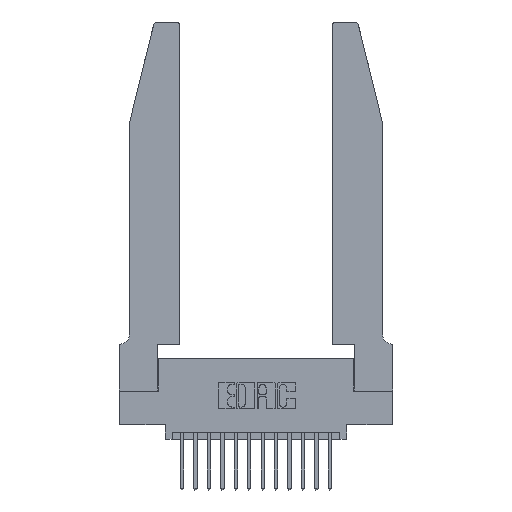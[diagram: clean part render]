
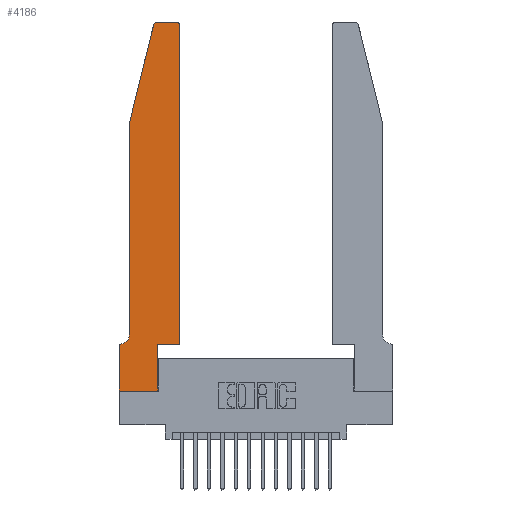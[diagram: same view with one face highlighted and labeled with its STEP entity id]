
A CAD part, top view. The second image highlights one B-rep face of the part: STEP entity #4186.
In plain terms, the highlighted planar face has unit normal (0, 0, 1).
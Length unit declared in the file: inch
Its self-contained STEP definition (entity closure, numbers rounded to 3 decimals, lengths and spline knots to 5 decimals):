
#68 = ORIENTED_EDGE ( 'NONE', *, *, #2993, .T. ) ;
#72 = CARTESIAN_POINT ( 'NONE',  ( 0.284, 2.75, 0.37 ) ) ;
#155 = EDGE_CURVE ( 'NONE', #11812, #13700, #17308, .T. ) ;
#1201 = EDGE_CURVE ( 'NONE', #9545, #7167, #5894, .T. ) ;
#1401 = LINE ( 'NONE', #8634, #16089 ) ;
#1418 = DIRECTION ( 'NONE',  ( 0., 0., 1. ) ) ;
#1608 = DIRECTION ( 'NONE',  ( 1., 0., 0. ) ) ;
#1954 = VECTOR ( 'NONE', #7813, 39.37008 ) ;
#1973 = VERTEX_POINT ( 'NONE', #15770 ) ;
#2091 = CARTESIAN_POINT ( 'NONE',  ( 0.0755, 0.35, 0.37 ) ) ;
#2262 = CARTESIAN_POINT ( 'NONE',  ( 0.4205, 2.75, 0.37 ) ) ;
#2316 = VERTEX_POINT ( 'NONE', #3792 ) ;
#2352 = CARTESIAN_POINT ( 'NONE',  ( 0.2865, 0., 0.37 ) ) ;
#2741 = DIRECTION ( 'NONE',  ( 0., 0., 1. ) ) ;
#2993 = EDGE_CURVE ( 'NONE', #6156, #1973, #8489, .T. ) ;
#3792 = CARTESIAN_POINT ( 'NONE',  ( 0.4505, 0.35, 0.37 ) ) ;
#3988 = VERTEX_POINT ( 'NONE', #17971 ) ;
#4166 = LINE ( 'NONE', #10574, #17501 ) ;
#4186 = ADVANCED_FACE ( 'NONE', ( #4870 ), #15073, .T. ) ;
#4292 = CARTESIAN_POINT ( 'NONE',  ( 0.4505, 2.72, 0.37 ) ) ;
#4484 = DIRECTION ( 'NONE',  ( 0., 0., -1. ) ) ;
#4489 = VECTOR ( 'NONE', #5891, 39.37008 ) ;
#4744 = AXIS2_PLACEMENT_3D ( 'NONE', #12536, #12012, #8576 ) ;
#4860 = ORIENTED_EDGE ( 'NONE', *, *, #15753, .T. ) ;
#4870 = FACE_OUTER_BOUND ( 'NONE', #14786, .T. ) ;
#5052 = ORIENTED_EDGE ( 'NONE', *, *, #17736, .T. ) ;
#5061 = VECTOR ( 'NONE', #9549, 39.37008 ) ;
#5888 = DIRECTION ( 'NONE',  ( -1., 0., 0. ) ) ;
#5891 = DIRECTION ( 'NONE',  ( 0., 1., 0. ) ) ;
#5894 = CIRCLE ( 'NONE', #4744, 0.03 ) ;
#5960 = VERTEX_POINT ( 'NONE', #13731 ) ;
#6041 = LINE ( 'NONE', #13011, #17624 ) ;
#6156 = VERTEX_POINT ( 'NONE', #72 ) ;
#6267 = EDGE_CURVE ( 'NONE', #13700, #17199, #4166, .T. ) ;
#6465 = DIRECTION ( 'NONE',  ( -1., 0., 0. ) ) ;
#6697 = CARTESIAN_POINT ( 'NONE',  ( 0., 0., 0.37 ) ) ;
#7167 = VERTEX_POINT ( 'NONE', #2262 ) ;
#7209 = CARTESIAN_POINT ( 'NONE',  ( 0.2865, 0.35, 0.37 ) ) ;
#7306 = DIRECTION ( 'NONE',  ( 0., 1., 0. ) ) ;
#7575 = CARTESIAN_POINT ( 'NONE',  ( 0.0755, 2., 0.37 ) ) ;
#7813 = DIRECTION ( 'NONE',  ( -1., 0., 0. ) ) ;
#8437 = LINE ( 'NONE', #7575, #14457 ) ;
#8489 = CIRCLE ( 'NONE', #11265, 0.03 ) ;
#8508 = ORIENTED_EDGE ( 'NONE', *, *, #6267, .T. ) ;
#8576 = DIRECTION ( 'NONE',  ( 1., 0., 0. ) ) ;
#8634 = CARTESIAN_POINT ( 'NONE',  ( 0.4505, 0.35, 0.37 ) ) ;
#8648 = ORIENTED_EDGE ( 'NONE', *, *, #13937, .T. ) ;
#8678 = CARTESIAN_POINT ( 'NONE',  ( 0., 0.35, 0.37 ) ) ;
#8901 = VERTEX_POINT ( 'NONE', #15929 ) ;
#8935 = DIRECTION ( 'NONE',  ( 1., 0., 0. ) ) ;
#9545 = VERTEX_POINT ( 'NONE', #4292 ) ;
#9549 = DIRECTION ( 'NONE',  ( 0., -1., 0. ) ) ;
#9565 = VERTEX_POINT ( 'NONE', #7209 ) ;
#9687 = EDGE_CURVE ( 'NONE', #5960, #3988, #8437, .T. ) ;
#9908 = CARTESIAN_POINT ( 'NONE',  ( 0.284, 2.72, 0.37 ) ) ;
#10032 = AXIS2_PLACEMENT_3D ( 'NONE', #10119, #4484, #5888 ) ;
#10039 = DIRECTION ( 'NONE',  ( 1., 0., 0. ) ) ;
#10119 = CARTESIAN_POINT ( 'NONE',  ( 0.0055, 0.42, 0.37 ) ) ;
#10574 = CARTESIAN_POINT ( 'NONE',  ( 0., 0., 0.37 ) ) ;
#10581 = ORIENTED_EDGE ( 'NONE', *, *, #12828, .T. ) ;
#10767 = ORIENTED_EDGE ( 'NONE', *, *, #155, .T. ) ;
#11215 = CARTESIAN_POINT ( 'NONE',  ( 0., 0.35, 0.37 ) ) ;
#11237 = EDGE_CURVE ( 'NONE', #8901, #11812, #17086, .T. ) ;
#11265 = AXIS2_PLACEMENT_3D ( 'NONE', #9908, #1418, #10039 ) ;
#11375 = ORIENTED_EDGE ( 'NONE', *, *, #9687, .T. ) ;
#11524 = ORIENTED_EDGE ( 'NONE', *, *, #11967, .T. ) ;
#11680 = LINE ( 'NONE', #14978, #16597 ) ;
#11690 = ORIENTED_EDGE ( 'NONE', *, *, #14386, .T. ) ;
#11812 = VERTEX_POINT ( 'NONE', #8678 ) ;
#11912 = CARTESIAN_POINT ( 'NONE',  ( 0., 0., 0.37 ) ) ;
#11967 = EDGE_CURVE ( 'NONE', #7167, #6156, #16563, .T. ) ;
#12012 = DIRECTION ( 'NONE',  ( 0., 0., 1. ) ) ;
#12536 = CARTESIAN_POINT ( 'NONE',  ( 0.4205, 2.72, 0.37 ) ) ;
#12808 = CARTESIAN_POINT ( 'NONE',  ( 0.2865, 0.35, 0.37 ) ) ;
#12828 = EDGE_CURVE ( 'NONE', #9565, #2316, #1401, .T. ) ;
#12940 = LINE ( 'NONE', #12808, #4489 ) ;
#13011 = CARTESIAN_POINT ( 'NONE',  ( 0.4505, 0.35, 0.37 ) ) ;
#13281 = DIRECTION ( 'NONE',  ( 0., -1., 0. ) ) ;
#13700 = VERTEX_POINT ( 'NONE', #6697 ) ;
#13731 = CARTESIAN_POINT ( 'NONE',  ( 0.0755, 2., 0.37 ) ) ;
#13937 = EDGE_CURVE ( 'NONE', #2316, #9545, #6041, .T. ) ;
#14218 = CIRCLE ( 'NONE', #10032, 0.07 ) ;
#14386 = EDGE_CURVE ( 'NONE', #17199, #9565, #12940, .T. ) ;
#14457 = VECTOR ( 'NONE', #13281, 39.37008 ) ;
#14786 = EDGE_LOOP ( 'NONE', ( #11524, #68, #5052, #11375, #4860, #16326, #10767, #8508, #11690, #10581, #8648, #17484 ) ) ;
#14978 = CARTESIAN_POINT ( 'NONE',  ( 0.0755, 2., 0.37 ) ) ;
#15073 = PLANE ( 'NONE',  #15625 ) ;
#15190 = CARTESIAN_POINT ( 'NONE',  ( 0.2605, 2.75, 0.37 ) ) ;
#15625 = AXIS2_PLACEMENT_3D ( 'NONE', #11215, #2741, #16903 ) ;
#15753 = EDGE_CURVE ( 'NONE', #3988, #8901, #14218, .T. ) ;
#15770 = CARTESIAN_POINT ( 'NONE',  ( 0.25487, 2.72718, 0.37 ) ) ;
#15929 = CARTESIAN_POINT ( 'NONE',  ( 0.0055, 0.35, 0.37 ) ) ;
#16089 = VECTOR ( 'NONE', #1608, 39.37008 ) ;
#16326 = ORIENTED_EDGE ( 'NONE', *, *, #11237, .T. ) ;
#16563 = LINE ( 'NONE', #15190, #17212 ) ;
#16597 = VECTOR ( 'NONE', #17862, 39.37008 ) ;
#16903 = DIRECTION ( 'NONE',  ( 1., 0., 0. ) ) ;
#17086 = LINE ( 'NONE', #2091, #1954 ) ;
#17199 = VERTEX_POINT ( 'NONE', #2352 ) ;
#17212 = VECTOR ( 'NONE', #6465, 39.37008 ) ;
#17308 = LINE ( 'NONE', #11912, #5061 ) ;
#17484 = ORIENTED_EDGE ( 'NONE', *, *, #1201, .T. ) ;
#17501 = VECTOR ( 'NONE', #8935, 39.37008 ) ;
#17624 = VECTOR ( 'NONE', #7306, 39.37008 ) ;
#17736 = EDGE_CURVE ( 'NONE', #1973, #5960, #11680, .T. ) ;
#17862 = DIRECTION ( 'NONE',  ( -0.239, -0.971, 0. ) ) ;
#17971 = CARTESIAN_POINT ( 'NONE',  ( 0.0755, 0.42, 0.37 ) ) ;
